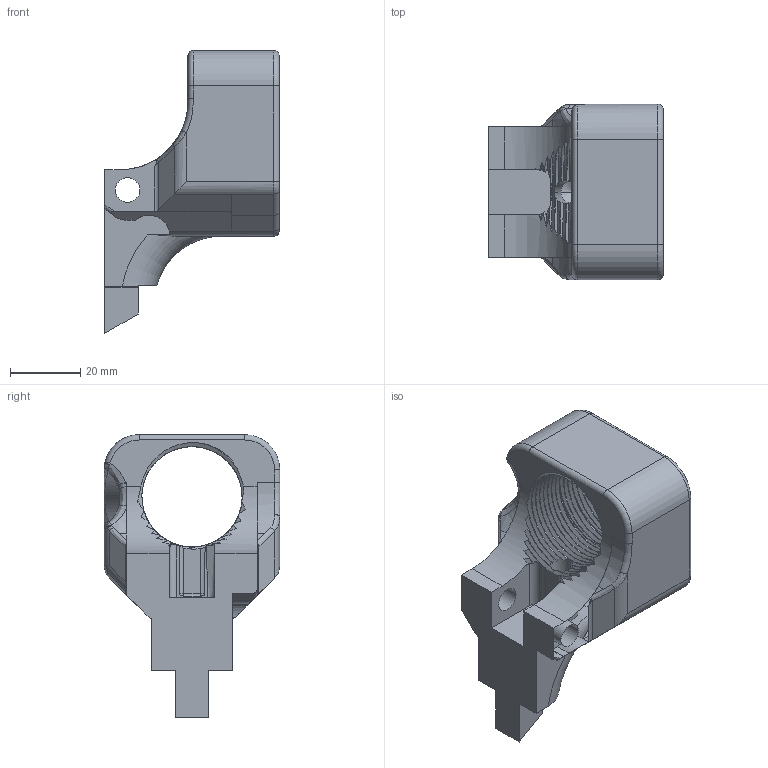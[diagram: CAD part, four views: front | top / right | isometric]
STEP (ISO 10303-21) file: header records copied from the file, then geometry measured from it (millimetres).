
FILE_DESCRIPTION (( 'STEP AP214' ), '1' );
FILE_NAME ('Phobos_V1.2_Rear.STEP', '2015-05-21T06:11:08', ( 'WarFairy' ), ( '' ), 'SwSTEP 2.0', 'SolidWorks 2015', '' );
FILE_SCHEMA (( 'AUTOMOTIVE_DESIGN' ));
Length unit declared in the file: inch
Products named in the file (1): Phobos_V1.2_Rear
Bounding box: 49.69 x 50 x 80.51 mm (x, y, z)
Volume: 65095.9 mm3; surface area: 17678.2 mm2
Topology: 1 solids, 1 shells, 215 faces, 635 edges, 417 vertices
Faces by surface type: cylinder 102, bspline 53, plane 43, torus 14, cone 2, sphere 1
Entity records: 20986 total; most frequent: CARTESIAN_POINT 16059, ORIENTED_EDGE 1262, DIRECTION 711, EDGE_CURVE 631, VERTEX_POINT 417, B_SPLINE_CURVE_WITH_KNOTS 299, AXIS2_PLACEMENT_3D 271, EDGE_LOOP 220
